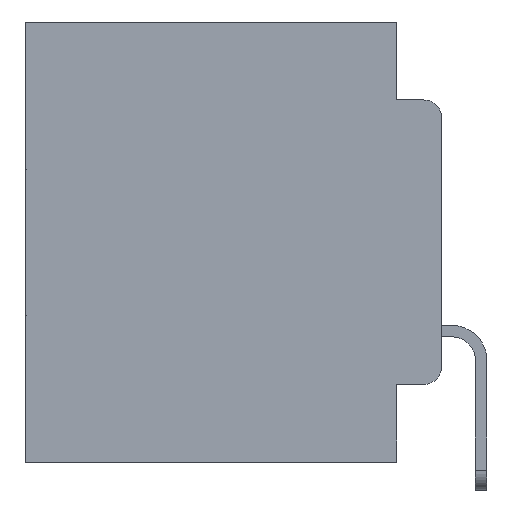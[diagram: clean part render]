
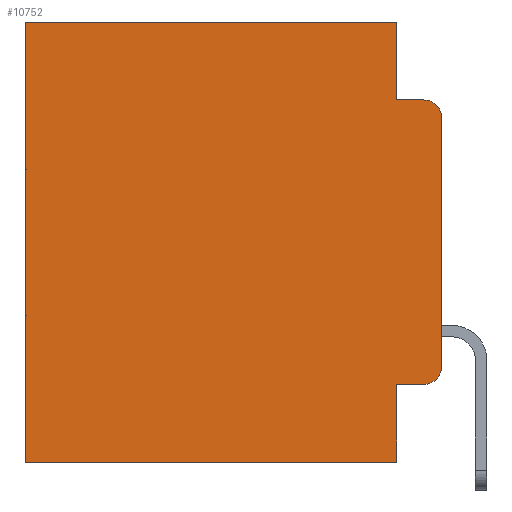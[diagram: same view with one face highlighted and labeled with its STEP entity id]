
A CAD part, left-side view. The second image highlights one B-rep face of the part: STEP entity #10752.
In plain terms, the highlighted planar face has unit normal (-1, 0, 0).
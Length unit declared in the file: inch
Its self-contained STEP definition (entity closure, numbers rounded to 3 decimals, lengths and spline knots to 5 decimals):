
#72 = EDGE_CURVE ( 'NONE', #27375, #18897, #21394, .T. ) ;
#397 = CARTESIAN_POINT ( 'NONE',  ( 0.298, 0.051, 0. ) ) ;
#405 = EDGE_CURVE ( 'NONE', #10529, #25374, #26814, .T. ) ;
#420 = DIRECTION ( 'NONE',  ( 0., 0., -1. ) ) ;
#448 = EDGE_CURVE ( 'NONE', #10529, #16187, #7327, .T. ) ;
#453 = EDGE_CURVE ( 'NONE', #9567, #16187, #1406, .T. ) ;
#459 = EDGE_CURVE ( 'NONE', #8332, #9567, #572, .T. ) ;
#462 = EDGE_CURVE ( 'NONE', #6354, #18897, #24290, .T. ) ;
#503 = EDGE_CURVE ( 'NONE', #1737, #27375, #23038, .T. ) ;
#505 = EDGE_CURVE ( 'NONE', #1737, #25336, #27765, .T. ) ;
#512 = EDGE_CURVE ( 'NONE', #25336, #25374, #17496, .T. ) ;
#572 = LINE ( 'NONE', #25844, #6551 ) ;
#1406 = LINE ( 'NONE', #21790, #18838 ) ;
#1737 = VERTEX_POINT ( 'NONE', #28305 ) ;
#2085 = DIRECTION ( 'NONE',  ( 0., 0., -1. ) ) ;
#2213 = VECTOR ( 'NONE', #25306, 39.37008 ) ;
#2395 = PLANE ( 'NONE',  #17468 ) ;
#2638 = LINE ( 'NONE', #21621, #14782 ) ;
#2764 = ORIENTED_EDGE ( 'NONE', *, *, #72, .F. ) ;
#2991 = ORIENTED_EDGE ( 'NONE', *, *, #12458, .T. ) ;
#3956 = ORIENTED_EDGE ( 'NONE', *, *, #462, .T. ) ;
#4046 = CARTESIAN_POINT ( 'NONE',  ( 0.298, 0.051, -0.0885 ) ) ;
#5418 = DIRECTION ( 'NONE',  ( 0., 0., -1. ) ) ;
#6354 = VERTEX_POINT ( 'NONE', #17074 ) ;
#6551 = VECTOR ( 'NONE', #13395, 39.37008 ) ;
#6669 = DIRECTION ( 'NONE',  ( 0., 1., 0. ) ) ;
#7141 = CARTESIAN_POINT ( 'NONE',  ( 0.298, 0.051, 0. ) ) ;
#7327 = CIRCLE ( 'NONE', #25998, 0.02 ) ;
#7450 = DIRECTION ( 'NONE',  ( 0., 0., -1. ) ) ;
#8049 = CARTESIAN_POINT ( 'NONE',  ( 0.298, 0.473, -0.5 ) ) ;
#8332 = VERTEX_POINT ( 'NONE', #397 ) ;
#8427 = DIRECTION ( 'NONE',  ( 0., -1., 0. ) ) ;
#9567 = VERTEX_POINT ( 'NONE', #4046 ) ;
#9609 = VECTOR ( 'NONE', #6669, 39.37008 ) ;
#10523 = CARTESIAN_POINT ( 'NONE',  ( 0.298, 0.051, -0.4115 ) ) ;
#10529 = VERTEX_POINT ( 'NONE', #22009 ) ;
#10752 = ADVANCED_FACE ( 'NONE', ( #11765 ), #2395, .F. ) ;
#10799 = VECTOR ( 'NONE', #13210, 39.37008 ) ;
#11765 = FACE_OUTER_BOUND ( 'NONE', #15011, .T. ) ;
#12287 = CARTESIAN_POINT ( 'NONE',  ( 0.298, 0.02, -0.3915 ) ) ;
#12312 = VECTOR ( 'NONE', #5418, 39.37008 ) ;
#12458 = EDGE_CURVE ( 'NONE', #8332, #6354, #2638, .T. ) ;
#12745 = AXIS2_PLACEMENT_3D ( 'NONE', #12287, #25198, #2085 ) ;
#13210 = DIRECTION ( 'NONE',  ( 0., -1., 0. ) ) ;
#13395 = DIRECTION ( 'NONE',  ( 0., 0., -1. ) ) ;
#13493 = DIRECTION ( 'NONE',  ( 0., 0., -1. ) ) ;
#13599 = ORIENTED_EDGE ( 'NONE', *, *, #503, .F. ) ;
#14782 = VECTOR ( 'NONE', #23657, 39.37008 ) ;
#15011 = EDGE_LOOP ( 'NONE', ( #19737, #21277, #23473, #26378, #2991, #3956, #2764, #13599, #16329, #16190 ) ) ;
#15066 = DIRECTION ( 'NONE',  ( -1., 0., 0. ) ) ;
#16187 = VERTEX_POINT ( 'NONE', #19883 ) ;
#16190 = ORIENTED_EDGE ( 'NONE', *, *, #512, .T. ) ;
#16329 = ORIENTED_EDGE ( 'NONE', *, *, #505, .T. ) ;
#16382 = CARTESIAN_POINT ( 'NONE',  ( 0.298, 0., -0.3915 ) ) ;
#17074 = CARTESIAN_POINT ( 'NONE',  ( 0.298, 0.473, 0. ) ) ;
#17468 = AXIS2_PLACEMENT_3D ( 'NONE', #18893, #20998, #7450 ) ;
#17496 = CIRCLE ( 'NONE', #12745, 0.02 ) ;
#18838 = VECTOR ( 'NONE', #8427, 39.37008 ) ;
#18893 = CARTESIAN_POINT ( 'NONE',  ( 0.298, 0., 0. ) ) ;
#18897 = VERTEX_POINT ( 'NONE', #8049 ) ;
#19737 = ORIENTED_EDGE ( 'NONE', *, *, #405, .F. ) ;
#19883 = CARTESIAN_POINT ( 'NONE',  ( 0.298, 0.02, -0.0885 ) ) ;
#20504 = CARTESIAN_POINT ( 'NONE',  ( 0.298, 0.02, -0.4115 ) ) ;
#20998 = DIRECTION ( 'NONE',  ( 1., 0., 0. ) ) ;
#21277 = ORIENTED_EDGE ( 'NONE', *, *, #448, .T. ) ;
#21394 = LINE ( 'NONE', #25816, #9609 ) ;
#21621 = CARTESIAN_POINT ( 'NONE',  ( 0.298, 0., 0. ) ) ;
#21790 = CARTESIAN_POINT ( 'NONE',  ( 0.298, 0.051, -0.0885 ) ) ;
#22009 = CARTESIAN_POINT ( 'NONE',  ( 0.298, 0., -0.1085 ) ) ;
#22797 = CARTESIAN_POINT ( 'NONE',  ( 0.298, 0., 0. ) ) ;
#23038 = LINE ( 'NONE', #7141, #12312 ) ;
#23473 = ORIENTED_EDGE ( 'NONE', *, *, #453, .F. ) ;
#23657 = DIRECTION ( 'NONE',  ( 0., 1., 0. ) ) ;
#23673 = VECTOR ( 'NONE', #13493, 39.37008 ) ;
#24290 = LINE ( 'NONE', #26414, #23673 ) ;
#25198 = DIRECTION ( 'NONE',  ( -1., 0., 0. ) ) ;
#25201 = CARTESIAN_POINT ( 'NONE',  ( 0.298, 0.051, -0.5 ) ) ;
#25306 = DIRECTION ( 'NONE',  ( 0., 0., -1. ) ) ;
#25336 = VERTEX_POINT ( 'NONE', #20504 ) ;
#25374 = VERTEX_POINT ( 'NONE', #16382 ) ;
#25816 = CARTESIAN_POINT ( 'NONE',  ( 0.298, 0., -0.5 ) ) ;
#25844 = CARTESIAN_POINT ( 'NONE',  ( 0.298, 0.051, 0. ) ) ;
#25998 = AXIS2_PLACEMENT_3D ( 'NONE', #27505, #15066, #420 ) ;
#26378 = ORIENTED_EDGE ( 'NONE', *, *, #459, .F. ) ;
#26414 = CARTESIAN_POINT ( 'NONE',  ( 0.298, 0.473, 0. ) ) ;
#26814 = LINE ( 'NONE', #22797, #2213 ) ;
#27375 = VERTEX_POINT ( 'NONE', #25201 ) ;
#27505 = CARTESIAN_POINT ( 'NONE',  ( 0.298, 0.02, -0.1085 ) ) ;
#27765 = LINE ( 'NONE', #10523, #10799 ) ;
#28305 = CARTESIAN_POINT ( 'NONE',  ( 0.298, 0.051, -0.4115 ) ) ;
